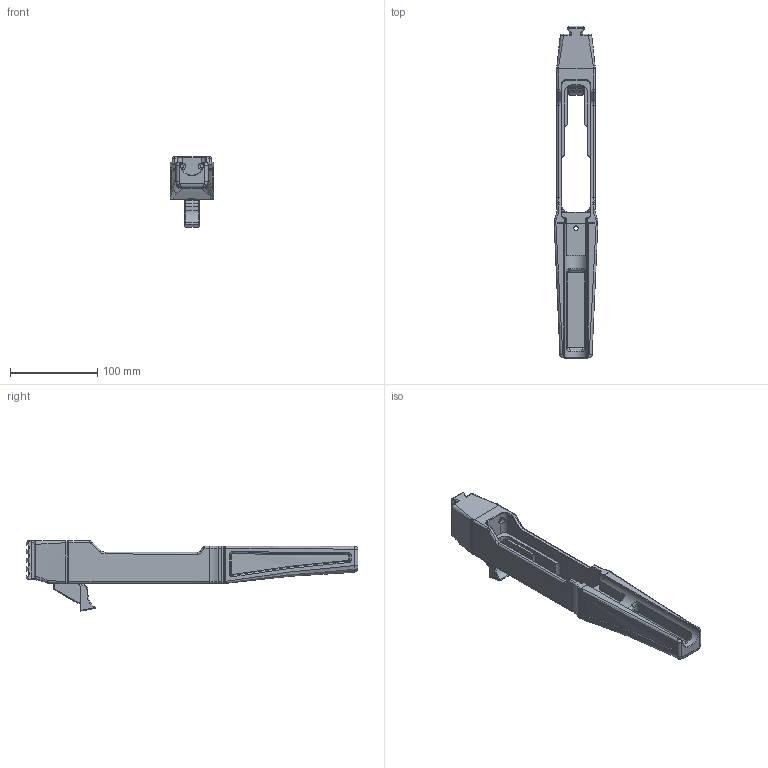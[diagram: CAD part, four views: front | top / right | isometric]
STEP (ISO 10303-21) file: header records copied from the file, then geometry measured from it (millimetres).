
FILE_DESCRIPTION(/* description */ (''),/* implementation_level */ '2;1');
FILE_NAME(/* name */ 'Full Chassis, Standard.step',/* time_stamp */ '2021-08-06T21:50:16-04:00',/* author */ (''),/* organization */ (''),/* preprocessor_version */ 'ST-DEVELOPER v18.1',/* originating_system */ 'Autodesk Translation Framework v10.9.0.1377',/* authorisation */ '');
FILE_SCHEMA (('AUTOMOTIVE_DESIGN { 1 0 10303 214 3 1 1 }'));
Length unit declared in the file: millimetre
Products named in the file (1): Full Chassis, Standard
Bounding box: 50.15 x 381.22 x 80.7 mm (x, y, z)
Volume: 333084.2 mm3; surface area: 95079.2 mm2
Topology: 3 solids, 4 shells, 692 faces, 1725 edges, 1039 vertices
Faces by surface type: plane 245, cylinder 199, bspline 157, torus 50, cone 31, sphere 10
Full cylindrical faces by diameter (mm): 3.8 x8, 5.3 x1, 6.097 x1, 8 x4, 9 x1, 20.317 x1, 23.683 x1
Entity records: 26167 total; most frequent: CARTESIAN_POINT 10522, ORIENTED_EDGE 3430, DIRECTION 2998, EDGE_CURVE 1715, AXIS2_PLACEMENT_3D 1097, VERTEX_POINT 1039, LINE 804, VECTOR 804
